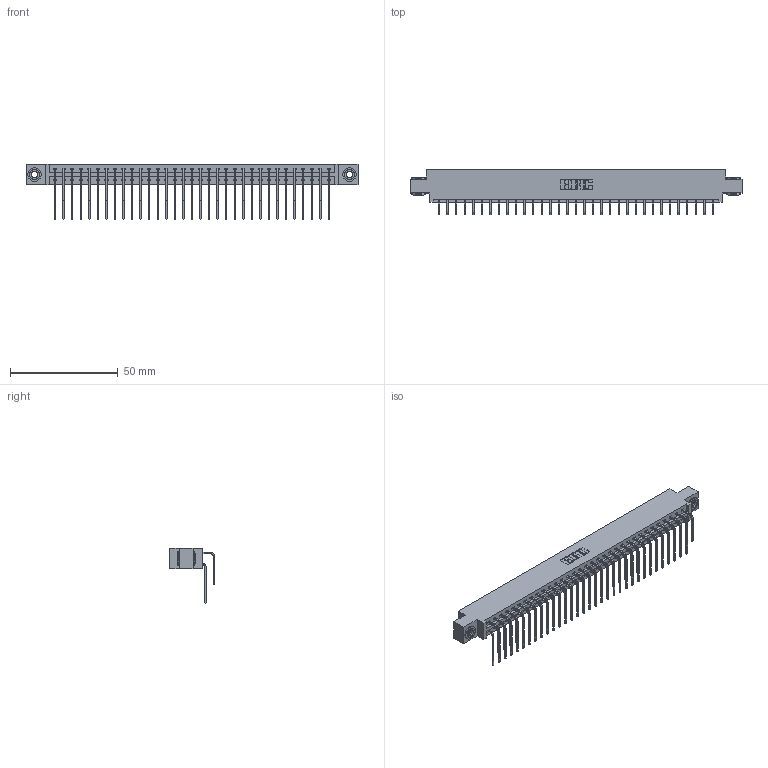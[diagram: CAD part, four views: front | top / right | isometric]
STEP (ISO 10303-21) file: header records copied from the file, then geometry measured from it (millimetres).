
FILE_DESCRIPTION (( 'STEP AP203' ), '1' );
FILE_NAME ('387-066-559-803.STEP', '2018-09-21T11:47:41', ( '' ), ( '' ), 'SwSTEP 2.0', 'SolidWorks 2016', '' );
FILE_SCHEMA (( 'CONFIG_CONTROL_DESIGN' ));
Length unit declared in the file: inch
Products named in the file (5): 337 Part_0.170 Offset - 0.156 Dia-TH; 345-292-001_558 559 Tail - 1; 345-292-001_559 Tail - 2; 345-250-002_345-250-002-102; 387-066-559-803
Assembly tree (69 placements, depth 2):
  387-066-559-803
    337 Part_0.170 Offset - 0.156 Dia-TH
    345-292-001_558 559 Tail - 1  x33
    345-292-001_559 Tail - 2  x33
    345-250-002_345-250-002-102  x2
Bounding box: 153.77 x 20.9 x 25.53 mm (x, y, z)
Volume: 16368.5 mm3; surface area: 20661.2 mm2
Topology: 69 solids, 69 shells, 3852 faces, 11421 edges, 7522 vertices
Faces by surface type: plane 2724, cylinder 1120, cone 8
Entity records: 29316 total; most frequent: CARTESIAN_POINT 4968, ORIENTED_EDGE 4846, DIRECTION 4257, EDGE_CURVE 2423, VECTOR 2231, LINE 2231, VERTEX_POINT 1610, AXIS2_PLACEMENT_3D 1013
